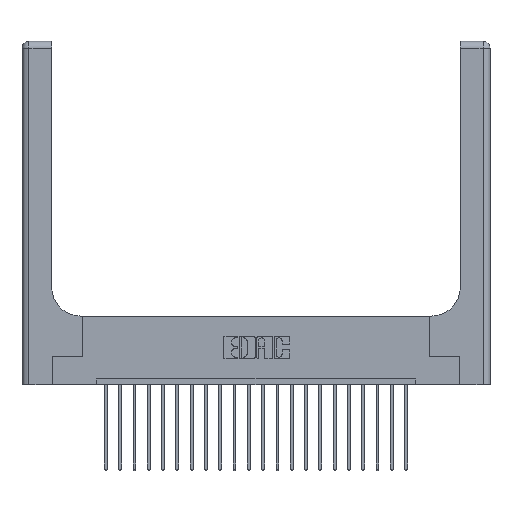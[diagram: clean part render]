
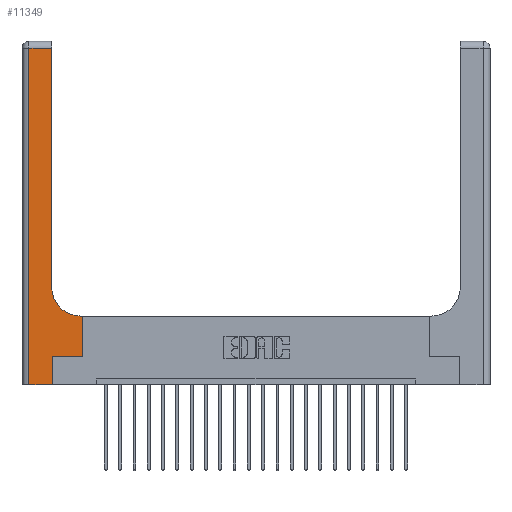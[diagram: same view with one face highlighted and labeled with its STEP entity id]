
A CAD part, top view. The second image highlights one B-rep face of the part: STEP entity #11349.
In plain terms, the highlighted planar face has unit normal (0, 0, 1).
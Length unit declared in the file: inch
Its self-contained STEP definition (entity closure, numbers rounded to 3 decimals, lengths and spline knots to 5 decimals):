
#97 = EDGE_CURVE ( 'NONE', #2909, #15743, #158, .T. ) ;
#158 = LINE ( 'NONE', #571, #19668 ) ;
#276 = CARTESIAN_POINT ( 'NONE',  ( 0.06, 2.94, 0.37 ) ) ;
#309 = LINE ( 'NONE', #17252, #13048 ) ;
#571 = CARTESIAN_POINT ( 'NONE',  ( 0., 0., 0.37 ) ) ;
#644 = VERTEX_POINT ( 'NONE', #276 ) ;
#1769 = CARTESIAN_POINT ( 'NONE',  ( 0., 2.94, 0.37 ) ) ;
#1780 = EDGE_LOOP ( 'NONE', ( #15145, #14504, #14350, #8466, #2451, #16301, #9371, #20335, #13060 ) ) ;
#1917 = CARTESIAN_POINT ( 'NONE',  ( 0.528, 0.6, 0.37 ) ) ;
#2301 = VECTOR ( 'NONE', #3498, 39.37008 ) ;
#2451 = ORIENTED_EDGE ( 'NONE', *, *, #8126, .T. ) ;
#2655 = VECTOR ( 'NONE', #4051, 39.37008 ) ;
#2909 = VERTEX_POINT ( 'NONE', #14675 ) ;
#2961 = CARTESIAN_POINT ( 'NONE',  ( 0.528, 0.25, 0.37 ) ) ;
#3498 = DIRECTION ( 'NONE',  ( 0., 1., 0. ) ) ;
#3790 = DIRECTION ( 'NONE',  ( 0., -1., 0. ) ) ;
#3836 = DIRECTION ( 'NONE',  ( 0., 0., -1. ) ) ;
#4051 = DIRECTION ( 'NONE',  ( 0., 1., 0. ) ) ;
#4325 = CARTESIAN_POINT ( 'NONE',  ( 0.265, 0., 0.37 ) ) ;
#4606 = DIRECTION ( 'NONE',  ( 0., 1., 0. ) ) ;
#5123 = AXIS2_PLACEMENT_3D ( 'NONE', #12880, #6032, #11152 ) ;
#5469 = DIRECTION ( 'NONE',  ( 1., 0., 0. ) ) ;
#5703 = EDGE_CURVE ( 'NONE', #11917, #10207, #20957, .T. ) ;
#6032 = DIRECTION ( 'NONE',  ( 0., 0., -1. ) ) ;
#6320 = CARTESIAN_POINT ( 'NONE',  ( 0.26, 2.94, 0.37 ) ) ;
#6362 = LINE ( 'NONE', #18797, #7118 ) ;
#6524 = LINE ( 'NONE', #15779, #2655 ) ;
#6941 = CARTESIAN_POINT ( 'NONE',  ( 0.51, 0.85, 0.37 ) ) ;
#7118 = VECTOR ( 'NONE', #3790, 39.37008 ) ;
#8077 = VERTEX_POINT ( 'NONE', #1917 ) ;
#8126 = EDGE_CURVE ( 'NONE', #15743, #11321, #20517, .T. ) ;
#8466 = ORIENTED_EDGE ( 'NONE', *, *, #97, .T. ) ;
#9371 = ORIENTED_EDGE ( 'NONE', *, *, #10414, .T. ) ;
#9916 = EDGE_CURVE ( 'NONE', #644, #2909, #6362, .T. ) ;
#10207 = VERTEX_POINT ( 'NONE', #13453 ) ;
#10329 = EDGE_CURVE ( 'NONE', #17013, #644, #16543, .T. ) ;
#10414 = EDGE_CURVE ( 'NONE', #14057, #8077, #17025, .T. ) ;
#11152 = DIRECTION ( 'NONE',  ( -1., 0., 0. ) ) ;
#11217 = PLANE ( 'NONE',  #5123 ) ;
#11321 = VERTEX_POINT ( 'NONE', #12049 ) ;
#11349 = ADVANCED_FACE ( 'NONE', ( #13369 ), #11217, .F. ) ;
#11917 = VERTEX_POINT ( 'NONE', #16240 ) ;
#12049 = CARTESIAN_POINT ( 'NONE',  ( 0.265, 0.25, 0.37 ) ) ;
#12083 = CARTESIAN_POINT ( 'NONE',  ( 0.265, 0., 0.37 ) ) ;
#12097 = EDGE_CURVE ( 'NONE', #10207, #17013, #6524, .T. ) ;
#12152 = EDGE_CURVE ( 'NONE', #8077, #11917, #14891, .T. ) ;
#12880 = CARTESIAN_POINT ( 'NONE',  ( 0., 3., 0.37 ) ) ;
#13048 = VECTOR ( 'NONE', #15468, 39.37008 ) ;
#13060 = ORIENTED_EDGE ( 'NONE', *, *, #5703, .T. ) ;
#13369 = FACE_OUTER_BOUND ( 'NONE', #1780, .T. ) ;
#13453 = CARTESIAN_POINT ( 'NONE',  ( 0.26, 0.85, 0.37 ) ) ;
#13580 = AXIS2_PLACEMENT_3D ( 'NONE', #6941, #3836, #5469 ) ;
#14057 = VERTEX_POINT ( 'NONE', #18841 ) ;
#14170 = DIRECTION ( 'NONE',  ( -1., 0., 0. ) ) ;
#14350 = ORIENTED_EDGE ( 'NONE', *, *, #9916, .T. ) ;
#14448 = VECTOR ( 'NONE', #4606, 39.37008 ) ;
#14504 = ORIENTED_EDGE ( 'NONE', *, *, #10329, .T. ) ;
#14675 = CARTESIAN_POINT ( 'NONE',  ( 0.06, 0., 0.37 ) ) ;
#14891 = LINE ( 'NONE', #20708, #21404 ) ;
#15145 = ORIENTED_EDGE ( 'NONE', *, *, #12097, .T. ) ;
#15468 = DIRECTION ( 'NONE',  ( 1., 0., 0. ) ) ;
#15743 = VERTEX_POINT ( 'NONE', #4325 ) ;
#15779 = CARTESIAN_POINT ( 'NONE',  ( 0.26, 3., 0.37 ) ) ;
#16240 = CARTESIAN_POINT ( 'NONE',  ( 0.51, 0.6, 0.37 ) ) ;
#16301 = ORIENTED_EDGE ( 'NONE', *, *, #19735, .T. ) ;
#16543 = LINE ( 'NONE', #1769, #20693 ) ;
#17013 = VERTEX_POINT ( 'NONE', #6320 ) ;
#17025 = LINE ( 'NONE', #2961, #14448 ) ;
#17214 = DIRECTION ( 'NONE',  ( -1., 0., 0. ) ) ;
#17252 = CARTESIAN_POINT ( 'NONE',  ( 0.265, 0.25, 0.37 ) ) ;
#18760 = DIRECTION ( 'NONE',  ( 1., 0., 0. ) ) ;
#18797 = CARTESIAN_POINT ( 'NONE',  ( 0.06, 3., 0.37 ) ) ;
#18841 = CARTESIAN_POINT ( 'NONE',  ( 0.528, 0.25, 0.37 ) ) ;
#19668 = VECTOR ( 'NONE', #18760, 39.37008 ) ;
#19735 = EDGE_CURVE ( 'NONE', #11321, #14057, #309, .T. ) ;
#20335 = ORIENTED_EDGE ( 'NONE', *, *, #12152, .T. ) ;
#20517 = LINE ( 'NONE', #12083, #2301 ) ;
#20693 = VECTOR ( 'NONE', #17214, 39.37008 ) ;
#20708 = CARTESIAN_POINT ( 'NONE',  ( 0.26, 0.6, 0.37 ) ) ;
#20957 = CIRCLE ( 'NONE', #13580, 0.25 ) ;
#21404 = VECTOR ( 'NONE', #14170, 39.37008 ) ;
